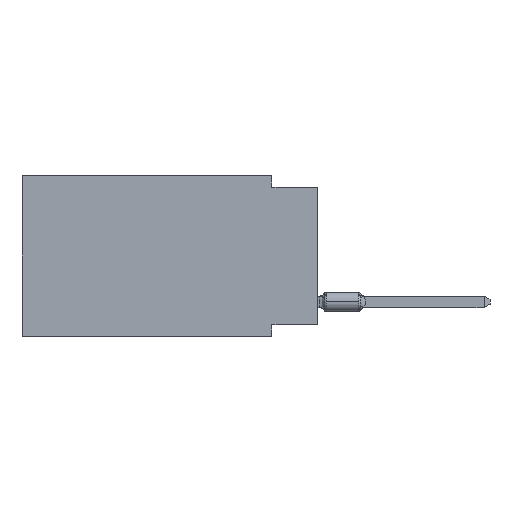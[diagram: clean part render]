
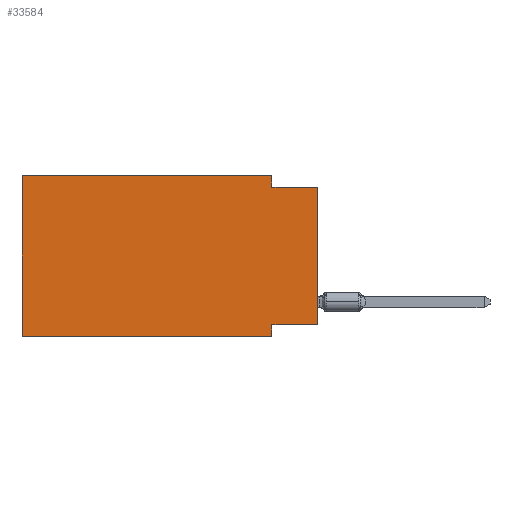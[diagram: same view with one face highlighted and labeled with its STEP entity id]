
A CAD part, left-side view. The second image highlights one B-rep face of the part: STEP entity #33584.
In plain terms, the highlighted planar face has unit normal (-1, 0, 0).
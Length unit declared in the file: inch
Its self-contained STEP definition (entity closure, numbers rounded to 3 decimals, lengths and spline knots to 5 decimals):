
#1462 = ORIENTED_EDGE ( 'NONE', *, *, #35953, .F. ) ;
#2121 = VECTOR ( 'NONE', #28451, 39.37008 ) ;
#2185 = ORIENTED_EDGE ( 'NONE', *, *, #29426, .F. ) ;
#3197 = DIRECTION ( 'NONE',  ( 0., 0., -1. ) ) ;
#3652 = DIRECTION ( 'NONE',  ( 1., 0., 0. ) ) ;
#4440 = CARTESIAN_POINT ( 'NONE',  ( 0., 0.1, -0.025 ) ) ;
#4621 = LINE ( 'NONE', #25517, #30192 ) ;
#5069 = ORIENTED_EDGE ( 'NONE', *, *, #35325, .T. ) ;
#6488 = ORIENTED_EDGE ( 'NONE', *, *, #12200, .F. ) ;
#7242 = CARTESIAN_POINT ( 'NONE',  ( 0., 0.645, -0.35 ) ) ;
#8127 = VERTEX_POINT ( 'NONE', #7242 ) ;
#8166 = ORIENTED_EDGE ( 'NONE', *, *, #8864, .T. ) ;
#8789 = CARTESIAN_POINT ( 'NONE',  ( 0., 0.1, 0. ) ) ;
#8864 = EDGE_CURVE ( 'NONE', #8127, #29250, #36929, .T. ) ;
#9245 = VERTEX_POINT ( 'NONE', #19384 ) ;
#10033 = FACE_OUTER_BOUND ( 'NONE', #16074, .T. ) ;
#10397 = CARTESIAN_POINT ( 'NONE',  ( 0., 0., 0. ) ) ;
#10737 = VERTEX_POINT ( 'NONE', #35476 ) ;
#11684 = VECTOR ( 'NONE', #16430, 39.37008 ) ;
#11898 = LINE ( 'NONE', #26033, #27829 ) ;
#12200 = EDGE_CURVE ( 'NONE', #8127, #30682, #22651, .T. ) ;
#14539 = CARTESIAN_POINT ( 'NONE',  ( 0., 0., -0.025 ) ) ;
#14708 = AXIS2_PLACEMENT_3D ( 'NONE', #24931, #3652, #21259 ) ;
#15770 = ORIENTED_EDGE ( 'NONE', *, *, #36598, .F. ) ;
#15866 = EDGE_CURVE ( 'NONE', #18423, #10737, #25387, .T. ) ;
#16074 = EDGE_LOOP ( 'NONE', ( #5069, #15770, #1462, #32111, #6488, #8166, #2185, #27298 ) ) ;
#16169 = VERTEX_POINT ( 'NONE', #4440 ) ;
#16430 = DIRECTION ( 'NONE',  ( 0., -1., 0. ) ) ;
#16543 = CARTESIAN_POINT ( 'NONE',  ( 0., 0.1, -0.35 ) ) ;
#17038 = CARTESIAN_POINT ( 'NONE',  ( 0., 0.645, 0. ) ) ;
#18423 = VERTEX_POINT ( 'NONE', #34938 ) ;
#19311 = LINE ( 'NONE', #36717, #22263 ) ;
#19384 = CARTESIAN_POINT ( 'NONE',  ( 0., 0.1, 0. ) ) ;
#19689 = LINE ( 'NONE', #10397, #33797 ) ;
#20454 = VERTEX_POINT ( 'NONE', #14539 ) ;
#21193 = DIRECTION ( 'NONE',  ( 0., 1., 0. ) ) ;
#21259 = DIRECTION ( 'NONE',  ( 0., 0., -1. ) ) ;
#21612 = VECTOR ( 'NONE', #21193, 39.37008 ) ;
#21634 = DIRECTION ( 'NONE',  ( 0., -1., 0. ) ) ;
#21831 = PLANE ( 'NONE',  #14708 ) ;
#22263 = VECTOR ( 'NONE', #21634, 39.37008 ) ;
#22405 = DIRECTION ( 'NONE',  ( 0., 0., 1. ) ) ;
#22651 = LINE ( 'NONE', #17038, #2121 ) ;
#23292 = DIRECTION ( 'NONE',  ( 0., 0., -1. ) ) ;
#24931 = CARTESIAN_POINT ( 'NONE',  ( 0., 0.645, 0. ) ) ;
#24980 = CARTESIAN_POINT ( 'NONE',  ( 0., 0.645, 0. ) ) ;
#25387 = LINE ( 'NONE', #34263, #21612 ) ;
#25517 = CARTESIAN_POINT ( 'NONE',  ( 0., 0., -0.025 ) ) ;
#26033 = CARTESIAN_POINT ( 'NONE',  ( 0., 0.1, -0.35 ) ) ;
#27298 = ORIENTED_EDGE ( 'NONE', *, *, #15866, .F. ) ;
#27829 = VECTOR ( 'NONE', #3197, 39.37008 ) ;
#28451 = DIRECTION ( 'NONE',  ( 0., 0., 1. ) ) ;
#29086 = LINE ( 'NONE', #8789, #33223 ) ;
#29250 = VERTEX_POINT ( 'NONE', #16543 ) ;
#29426 = EDGE_CURVE ( 'NONE', #10737, #29250, #11898, .T. ) ;
#30192 = VECTOR ( 'NONE', #37118, 39.37008 ) ;
#30682 = VERTEX_POINT ( 'NONE', #24980 ) ;
#32111 = ORIENTED_EDGE ( 'NONE', *, *, #38118, .F. ) ;
#33223 = VECTOR ( 'NONE', #23292, 39.37008 ) ;
#33584 = ADVANCED_FACE ( 'NONE', ( #10033 ), #21831, .F. ) ;
#33797 = VECTOR ( 'NONE', #22405, 39.37008 ) ;
#34263 = CARTESIAN_POINT ( 'NONE',  ( 0., 0., -0.325 ) ) ;
#34938 = CARTESIAN_POINT ( 'NONE',  ( 0., 0., -0.325 ) ) ;
#35325 = EDGE_CURVE ( 'NONE', #18423, #20454, #19689, .T. ) ;
#35476 = CARTESIAN_POINT ( 'NONE',  ( 0., 0.1, -0.325 ) ) ;
#35953 = EDGE_CURVE ( 'NONE', #9245, #16169, #29086, .T. ) ;
#36549 = CARTESIAN_POINT ( 'NONE',  ( 0., 0.645, -0.35 ) ) ;
#36598 = EDGE_CURVE ( 'NONE', #16169, #20454, #4621, .T. ) ;
#36717 = CARTESIAN_POINT ( 'NONE',  ( 0., 0.645, 0. ) ) ;
#36929 = LINE ( 'NONE', #36549, #11684 ) ;
#37118 = DIRECTION ( 'NONE',  ( 0., -1., 0. ) ) ;
#38118 = EDGE_CURVE ( 'NONE', #30682, #9245, #19311, .T. ) ;
